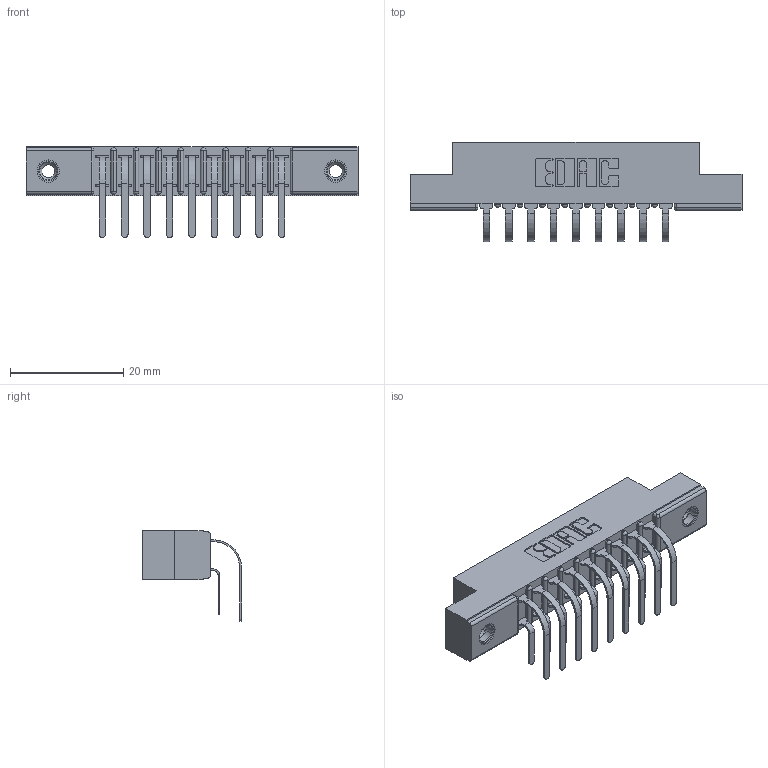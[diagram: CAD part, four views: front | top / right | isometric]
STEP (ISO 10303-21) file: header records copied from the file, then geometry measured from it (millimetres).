
FILE_DESCRIPTION (( 'STEP AP203' ), '1' );
FILE_NAME ('357-018-459-208.STEP', '2022-07-08T01:07:07', ( '' ), ( '' ), 'SwSTEP 2.0', 'SolidWorks 2020', '' );
FILE_SCHEMA (( 'CONFIG_CONTROL_DESIGN' ));
Length unit declared in the file: inch
Products named in the file (5): 345-250-001_345-250-003-102; 307 Part_.156 Dia Mounting Holes; 357-018-459-208; 307-290-001_559 - 2 (Single); 307-290-001_558 559 - 1 (Single)
Assembly tree (21 placements, depth 2):
  357-018-459-208
    307 Part_.156 Dia Mounting Holes
    307-290-001_558 559 - 1 (Single)  x9
    307-290-001_559 - 2 (Single)  x9
    345-250-001_345-250-003-102  x2
Bounding box: 58.67 x 17.51 x 16.08 mm (x, y, z)
Volume: 3900.6 mm3; surface area: 6609.6 mm2
Topology: 21 solids, 21 shells, 1088 faces, 3015 edges, 1950 vertices
Faces by surface type: plane 696, cylinder 356, sphere 20, cone 12, torus 4
Entity records: 14704 total; most frequent: CARTESIAN_POINT 2402, DIRECTION 2375, ORIENTED_EDGE 2370, EDGE_CURVE 1185, LINE 893, VECTOR 893, VERTEX_POINT 768, AXIS2_PLACEMENT_3D 741
